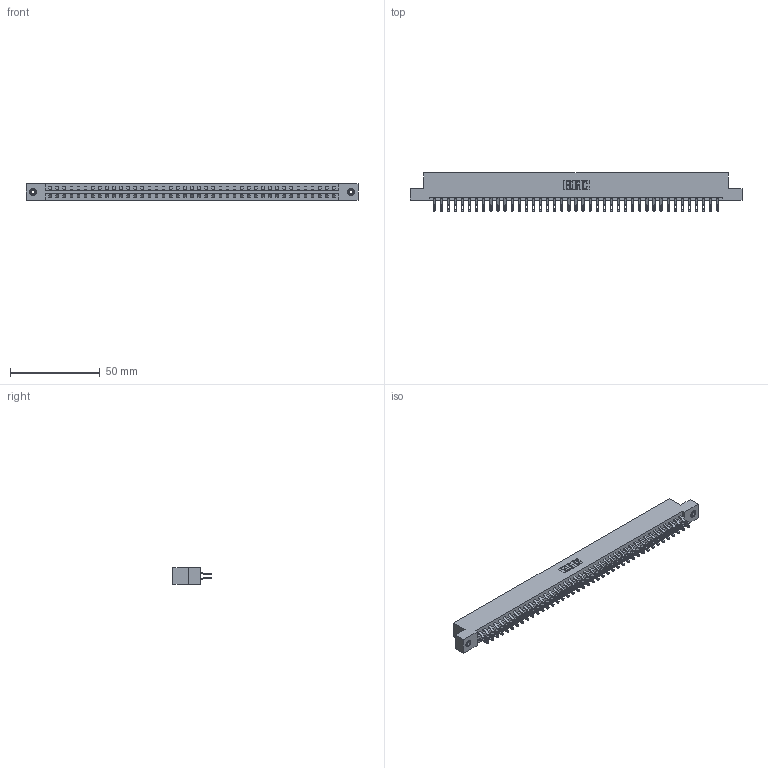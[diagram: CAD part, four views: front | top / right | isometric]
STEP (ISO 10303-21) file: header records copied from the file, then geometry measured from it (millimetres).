
FILE_DESCRIPTION (( 'STEP AP203' ), '1' );
FILE_NAME ('337-082-555-208.STEP', '2019-10-10T13:18:06', ( '' ), ( '' ), 'SwSTEP 2.0', 'SolidWorks 2016', '' );
FILE_SCHEMA (( 'CONFIG_CONTROL_DESIGN' ));
Length unit declared in the file: inch
Products named in the file (4): 345-292-001_555 Tail; 337 Part_Flush Mounting Lugs - 0.156 Dia-TI; 337-082-555-208; 345-250-001_345-250-003-102
Assembly tree (85 placements, depth 2):
  337-082-555-208
    337 Part_Flush Mounting Lugs - 0.156 Dia-TI
    345-292-001_555 Tail  x82
    345-250-001_345-250-003-102  x2
Bounding box: 185.47 x 21.47 x 9.4 mm (x, y, z)
Volume: 19764.4 mm3; surface area: 23254.2 mm2
Topology: 85 solids, 85 shells, 5094 faces, 15945 edges, 10622 vertices
Faces by surface type: plane 3054, cylinder 2024, cone 12, torus 4
Entity records: 33430 total; most frequent: CARTESIAN_POINT 5647, ORIENTED_EDGE 5546, DIRECTION 4807, EDGE_CURVE 2773, VECTOR 2605, LINE 2605, VERTEX_POINT 1844, AXIS2_PLACEMENT_3D 1101
